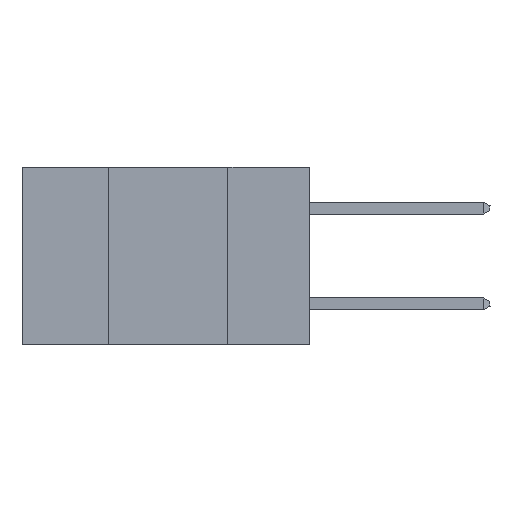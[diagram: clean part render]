
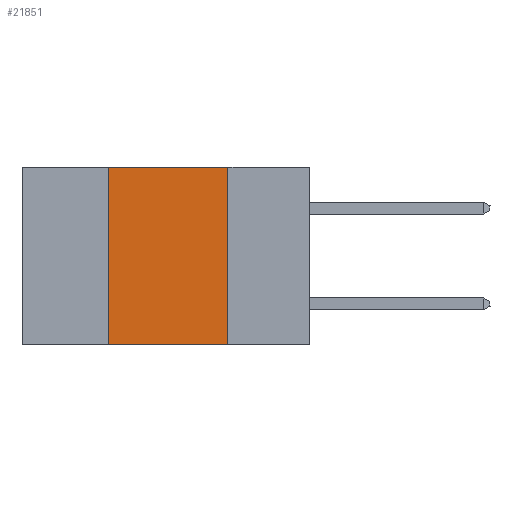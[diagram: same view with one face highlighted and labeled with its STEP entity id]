
A CAD part, left-side view. The second image highlights one B-rep face of the part: STEP entity #21851.
In plain terms, the highlighted planar face has unit normal (-1, 0, 0).
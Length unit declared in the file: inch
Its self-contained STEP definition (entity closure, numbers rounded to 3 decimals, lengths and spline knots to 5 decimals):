
#1167 = CARTESIAN_POINT ( 'NONE',  ( 0., 0.6, 0. ) ) ;
#1546 = LINE ( 'NONE', #5104, #20981 ) ;
#2649 = CARTESIAN_POINT ( 'NONE',  ( 0., 0.17, -0.37 ) ) ;
#2923 = DIRECTION ( 'NONE',  ( 0., 0., -1. ) ) ;
#2964 = LINE ( 'NONE', #27742, #32126 ) ;
#4396 = VECTOR ( 'NONE', #16962, 39.37008 ) ;
#4533 = VERTEX_POINT ( 'NONE', #29811 ) ;
#5104 = CARTESIAN_POINT ( 'NONE',  ( 0., 0.6, 0. ) ) ;
#5225 = DIRECTION ( 'NONE',  ( 0., -1., 0. ) ) ;
#8759 = EDGE_CURVE ( 'NONE', #10565, #4533, #1546, .T. ) ;
#10565 = VERTEX_POINT ( 'NONE', #17559 ) ;
#11548 = EDGE_LOOP ( 'NONE', ( #23825, #14446, #23270, #14094 ) ) ;
#11596 = DIRECTION ( 'NONE',  ( 0., -1., 0. ) ) ;
#11811 = DIRECTION ( 'NONE',  ( 0., 0., -1. ) ) ;
#13607 = EDGE_CURVE ( 'NONE', #4533, #19673, #26751, .T. ) ;
#14094 = ORIENTED_EDGE ( 'NONE', *, *, #29567, .T. ) ;
#14446 = ORIENTED_EDGE ( 'NONE', *, *, #8759, .F. ) ;
#16013 = FACE_OUTER_BOUND ( 'NONE', #11548, .T. ) ;
#16962 = DIRECTION ( 'NONE',  ( 0., 0., 1. ) ) ;
#17559 = CARTESIAN_POINT ( 'NONE',  ( 0., 0.42, 0. ) ) ;
#19673 = VERTEX_POINT ( 'NONE', #2649 ) ;
#19929 = DIRECTION ( 'NONE',  ( 1., 0., 0. ) ) ;
#20829 = VECTOR ( 'NONE', #2923, 39.37008 ) ;
#20981 = VECTOR ( 'NONE', #5225, 39.37008 ) ;
#21662 = LINE ( 'NONE', #22235, #4396 ) ;
#21851 = ADVANCED_FACE ( 'NONE', ( #16013 ), #33164, .F. ) ;
#22235 = CARTESIAN_POINT ( 'NONE',  ( 0., 0.42, 0. ) ) ;
#23270 = ORIENTED_EDGE ( 'NONE', *, *, #33535, .F. ) ;
#23825 = ORIENTED_EDGE ( 'NONE', *, *, #13607, .F. ) ;
#24383 = CARTESIAN_POINT ( 'NONE',  ( 0., 0.17, 0. ) ) ;
#24385 = VERTEX_POINT ( 'NONE', #24721 ) ;
#24721 = CARTESIAN_POINT ( 'NONE',  ( 0., 0.42, -0.37 ) ) ;
#26751 = LINE ( 'NONE', #24383, #20829 ) ;
#27742 = CARTESIAN_POINT ( 'NONE',  ( 0., 0.6, -0.37 ) ) ;
#29567 = EDGE_CURVE ( 'NONE', #24385, #19673, #2964, .T. ) ;
#29811 = CARTESIAN_POINT ( 'NONE',  ( 0., 0.17, 0. ) ) ;
#32126 = VECTOR ( 'NONE', #11596, 39.37008 ) ;
#33164 = PLANE ( 'NONE',  #33665 ) ;
#33535 = EDGE_CURVE ( 'NONE', #24385, #10565, #21662, .T. ) ;
#33665 = AXIS2_PLACEMENT_3D ( 'NONE', #1167, #19929, #11811 ) ;
